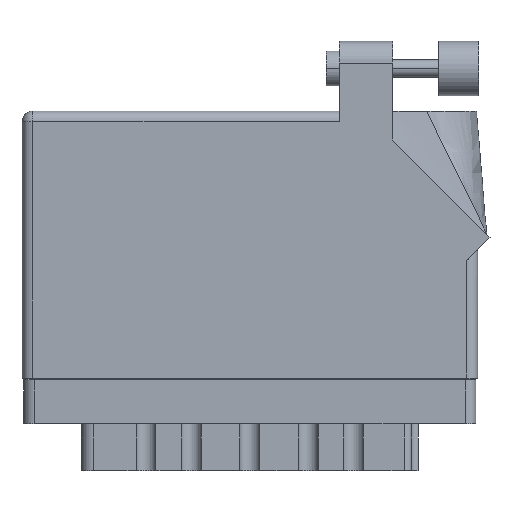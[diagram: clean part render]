
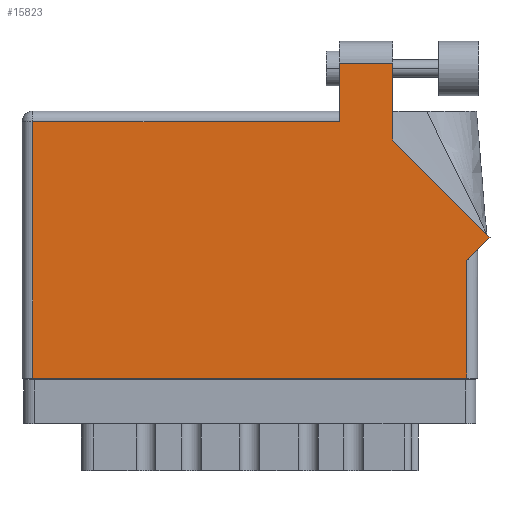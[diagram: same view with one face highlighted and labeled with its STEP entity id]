
A CAD part, front view. The second image highlights one B-rep face of the part: STEP entity #15823.
In plain terms, the highlighted face is planar.
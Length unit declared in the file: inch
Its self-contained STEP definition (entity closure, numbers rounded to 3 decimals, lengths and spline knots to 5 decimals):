
#79 = CARTESIAN_POINT ( 'NONE',  ( 1.819, 1.805, 0. ) ) ;
#202 = CARTESIAN_POINT ( 'NONE',  ( 2.55, 0.737, 0. ) ) ;
#952 = CARTESIAN_POINT ( 'NONE',  ( 0.062, 0., 0. ) ) ;
#1738 = DIRECTION ( 'NONE',  ( -0.707, 0.707, 0. ) ) ;
#1982 = VERTEX_POINT ( 'NONE', #5346 ) ;
#1998 = VERTEX_POINT ( 'NONE', #22443 ) ;
#2076 = VECTOR ( 'NONE', #25204, 39.37008 ) ;
#3426 = LINE ( 'NONE', #7496, #37140 ) ;
#3672 = ORIENTED_EDGE ( 'NONE', *, *, #17403, .T. ) ;
#5346 = CARTESIAN_POINT ( 'NONE',  ( 1.819, 1.805, 0. ) ) ;
#6227 = ORIENTED_EDGE ( 'NONE', *, *, #11876, .T. ) ;
#6767 = ORIENTED_EDGE ( 'NONE', *, *, #26125, .T. ) ;
#7496 = CARTESIAN_POINT ( 'NONE',  ( 1.819, 1.53, 0. ) ) ;
#8001 = EDGE_CURVE ( 'NONE', #1982, #15246, #3426, .T. ) ;
#8431 = ORIENTED_EDGE ( 'NONE', *, *, #36610, .T. ) ;
#10618 = DIRECTION ( 'NONE',  ( 0., 1., 0. ) ) ;
#11876 = EDGE_CURVE ( 'NONE', #38157, #40303, #15993, .T. ) ;
#13393 = LINE ( 'NONE', #952, #2076 ) ;
#13501 = DIRECTION ( 'NONE',  ( -1., 0., 0. ) ) ;
#13866 = CARTESIAN_POINT ( 'NONE',  ( 1.819, 1.468, 0. ) ) ;
#14221 = VECTOR ( 'NONE', #27316, 39.37008 ) ;
#14723 = ORIENTED_EDGE ( 'NONE', *, *, #39936, .T. ) ;
#15215 = FACE_OUTER_BOUND ( 'NONE', #23231, .T. ) ;
#15246 = VERTEX_POINT ( 'NONE', #13866 ) ;
#15625 = VECTOR ( 'NONE', #43239, 39.37008 ) ;
#15823 = ADVANCED_FACE ( 'NONE', ( #15215 ), #40353, .F. ) ;
#15993 = LINE ( 'NONE', #38409, #19789 ) ;
#17403 = EDGE_CURVE ( 'NONE', #20376, #37742, #36378, .T. ) ;
#18221 = CARTESIAN_POINT ( 'NONE',  ( 2.126, 1.805, 0. ) ) ;
#18897 = LINE ( 'NONE', #43147, #21609 ) ;
#19317 = LINE ( 'NONE', #79, #22609 ) ;
#19392 = EDGE_CURVE ( 'NONE', #31474, #20376, #22127, .T. ) ;
#19789 = VECTOR ( 'NONE', #34436, 39.37008 ) ;
#19930 = EDGE_CURVE ( 'NONE', #37742, #1982, #19317, .T. ) ;
#20376 = VERTEX_POINT ( 'NONE', #26845 ) ;
#21521 = AXIS2_PLACEMENT_3D ( 'NONE', #36238, #43252, #44002 ) ;
#21609 = VECTOR ( 'NONE', #39190, 39.37008 ) ;
#22127 = LINE ( 'NONE', #32713, #27062 ) ;
#22443 = CARTESIAN_POINT ( 'NONE',  ( 0.062, 1.468, 0. ) ) ;
#22508 = ORIENTED_EDGE ( 'NONE', *, *, #19930, .T. ) ;
#22609 = VECTOR ( 'NONE', #13501, 39.37008 ) ;
#23231 = EDGE_LOOP ( 'NONE', ( #3672, #22508, #23413, #44436, #8431, #6227, #14723, #6767, #43989 ) ) ;
#23413 = ORIENTED_EDGE ( 'NONE', *, *, #8001, .T. ) ;
#24971 = DIRECTION ( 'NONE',  ( 0., -1., 0. ) ) ;
#25204 = DIRECTION ( 'NONE',  ( 0., -1., 0. ) ) ;
#26125 = EDGE_CURVE ( 'NONE', #26964, #31474, #27299, .T. ) ;
#26845 = CARTESIAN_POINT ( 'NONE',  ( 2.126, 1.36442, 0. ) ) ;
#26964 = VERTEX_POINT ( 'NONE', #42919 ) ;
#27062 = VECTOR ( 'NONE', #1738, 39.37008 ) ;
#27299 = LINE ( 'NONE', #37960, #14221 ) ;
#27316 = DIRECTION ( 'NONE',  ( 0.707, 0.707, 0. ) ) ;
#28444 = VECTOR ( 'NONE', #10618, 39.37008 ) ;
#31474 = VERTEX_POINT ( 'NONE', #43453 ) ;
#31697 = LINE ( 'NONE', #202, #28444 ) ;
#32713 = CARTESIAN_POINT ( 'NONE',  ( 2.68271, 0.80771, 0. ) ) ;
#34436 = DIRECTION ( 'NONE',  ( 1., 0., 0. ) ) ;
#36238 = CARTESIAN_POINT ( 'NONE',  ( 0., 1.53, 0. ) ) ;
#36378 = LINE ( 'NONE', #36521, #15625 ) ;
#36521 = CARTESIAN_POINT ( 'NONE',  ( 2.126, 1.36442, 0. ) ) ;
#36610 = EDGE_CURVE ( 'NONE', #1998, #38157, #13393, .T. ) ;
#37140 = VECTOR ( 'NONE', #24971, 39.37008 ) ;
#37255 = EDGE_CURVE ( 'NONE', #15246, #1998, #18897, .T. ) ;
#37742 = VERTEX_POINT ( 'NONE', #18221 ) ;
#37960 = CARTESIAN_POINT ( 'NONE',  ( 2.612, 0.737, 0. ) ) ;
#38157 = VERTEX_POINT ( 'NONE', #42152 ) ;
#38409 = CARTESIAN_POINT ( 'NONE',  ( 0., 0., 0. ) ) ;
#39190 = DIRECTION ( 'NONE',  ( -1., 0., 0. ) ) ;
#39936 = EDGE_CURVE ( 'NONE', #40303, #26964, #31697, .T. ) ;
#40303 = VERTEX_POINT ( 'NONE', #44104 ) ;
#40353 = PLANE ( 'NONE',  #21521 ) ;
#42152 = CARTESIAN_POINT ( 'NONE',  ( 0.062, 0., 0. ) ) ;
#42919 = CARTESIAN_POINT ( 'NONE',  ( 2.55, 0.675, 0. ) ) ;
#43147 = CARTESIAN_POINT ( 'NONE',  ( 0., 1.468, 0. ) ) ;
#43239 = DIRECTION ( 'NONE',  ( 0., 1., 0. ) ) ;
#43252 = DIRECTION ( 'NONE',  ( 0., 0., -1. ) ) ;
#43453 = CARTESIAN_POINT ( 'NONE',  ( 2.68271, 0.80771, 0. ) ) ;
#43989 = ORIENTED_EDGE ( 'NONE', *, *, #19392, .T. ) ;
#44002 = DIRECTION ( 'NONE',  ( -1., 0., 0. ) ) ;
#44104 = CARTESIAN_POINT ( 'NONE',  ( 2.55, 0., 0. ) ) ;
#44436 = ORIENTED_EDGE ( 'NONE', *, *, #37255, .T. ) ;
